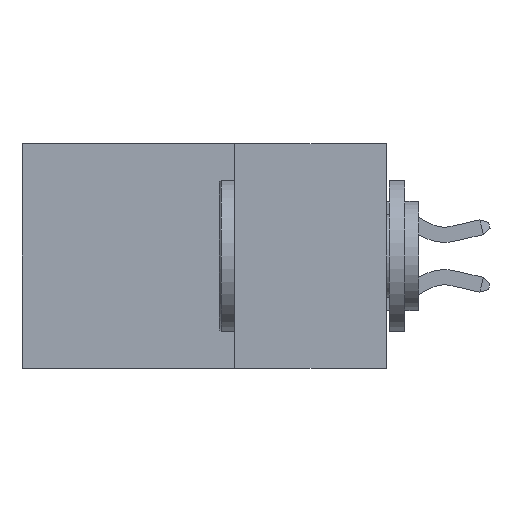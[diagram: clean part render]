
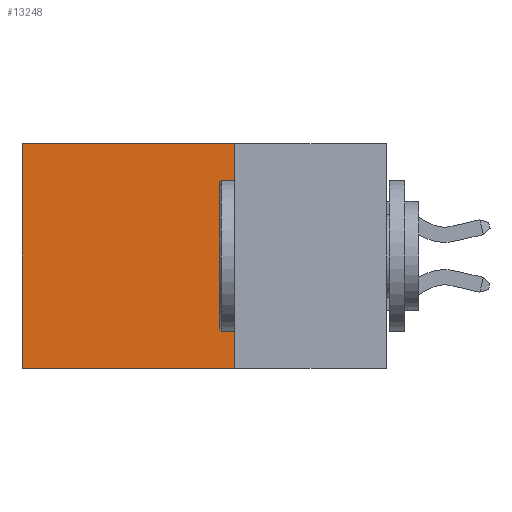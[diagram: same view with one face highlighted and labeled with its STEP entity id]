
A CAD part, left-side view. The second image highlights one B-rep face of the part: STEP entity #13248.
In plain terms, the highlighted planar face has unit normal (-1, 0, 0).
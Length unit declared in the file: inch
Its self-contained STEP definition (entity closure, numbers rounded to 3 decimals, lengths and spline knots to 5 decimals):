
#138 = CARTESIAN_POINT ( 'NONE',  ( 0.298, 0.6, -0.37 ) ) ;
#331 = CARTESIAN_POINT ( 'NONE',  ( 0.298, 0.25, 0. ) ) ;
#627 = PLANE ( 'NONE',  #8087 ) ;
#668 = DIRECTION ( 'NONE',  ( 0., 1., 0. ) ) ;
#942 = ORIENTED_EDGE ( 'NONE', *, *, #9586, .T. ) ;
#1456 = DIRECTION ( 'NONE',  ( 0., 0., -1. ) ) ;
#1566 = LINE ( 'NONE', #14073, #6761 ) ;
#1953 = EDGE_CURVE ( 'NONE', #2640, #8834, #13391, .T. ) ;
#2006 = ORIENTED_EDGE ( 'NONE', *, *, #8449, .F. ) ;
#2640 = VERTEX_POINT ( 'NONE', #6751 ) ;
#3274 = FACE_OUTER_BOUND ( 'NONE', #3407, .T. ) ;
#3407 = EDGE_LOOP ( 'NONE', ( #942, #2006, #4837, #13414 ) ) ;
#4837 = ORIENTED_EDGE ( 'NONE', *, *, #5470, .F. ) ;
#5470 = EDGE_CURVE ( 'NONE', #2640, #6460, #13987, .T. ) ;
#5976 = CARTESIAN_POINT ( 'NONE',  ( 0.298, 0.25, -0.37 ) ) ;
#6460 = VERTEX_POINT ( 'NONE', #7750 ) ;
#6751 = CARTESIAN_POINT ( 'NONE',  ( 0.298, 0.25, 0. ) ) ;
#6761 = VECTOR ( 'NONE', #14030, 39.37008 ) ;
#7336 = VECTOR ( 'NONE', #668, 39.37008 ) ;
#7750 = CARTESIAN_POINT ( 'NONE',  ( 0.298, 0.25, -0.37 ) ) ;
#7813 = VECTOR ( 'NONE', #11788, 39.37008 ) ;
#7942 = VERTEX_POINT ( 'NONE', #138 ) ;
#8087 = AXIS2_PLACEMENT_3D ( 'NONE', #331, #8515, #1456 ) ;
#8261 = VECTOR ( 'NONE', #14723, 39.37008 ) ;
#8449 = EDGE_CURVE ( 'NONE', #6460, #7942, #13563, .T. ) ;
#8515 = DIRECTION ( 'NONE',  ( 1., 0., 0. ) ) ;
#8834 = VERTEX_POINT ( 'NONE', #13642 ) ;
#9586 = EDGE_CURVE ( 'NONE', #8834, #7942, #1566, .T. ) ;
#10217 = CARTESIAN_POINT ( 'NONE',  ( 0.298, 0.25, 0. ) ) ;
#11453 = CARTESIAN_POINT ( 'NONE',  ( 0.298, 0.25, 0. ) ) ;
#11788 = DIRECTION ( 'NONE',  ( 0., 0., -1. ) ) ;
#13248 = ADVANCED_FACE ( 'NONE', ( #3274 ), #627, .F. ) ;
#13391 = LINE ( 'NONE', #11453, #8261 ) ;
#13414 = ORIENTED_EDGE ( 'NONE', *, *, #1953, .T. ) ;
#13563 = LINE ( 'NONE', #5976, #7336 ) ;
#13642 = CARTESIAN_POINT ( 'NONE',  ( 0.298, 0.6, 0. ) ) ;
#13987 = LINE ( 'NONE', #10217, #7813 ) ;
#14030 = DIRECTION ( 'NONE',  ( 0., 0., -1. ) ) ;
#14073 = CARTESIAN_POINT ( 'NONE',  ( 0.298, 0.6, 0. ) ) ;
#14723 = DIRECTION ( 'NONE',  ( 0., 1., 0. ) ) ;
